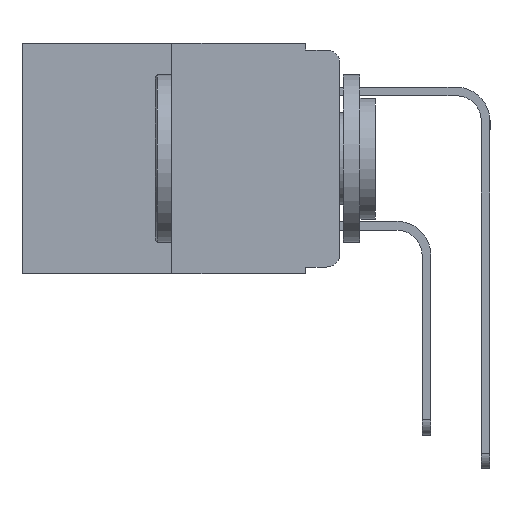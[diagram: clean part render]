
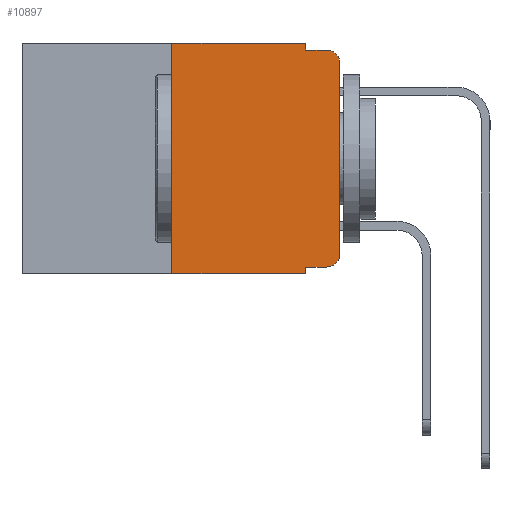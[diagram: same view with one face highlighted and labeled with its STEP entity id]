
A CAD part, left-side view. The second image highlights one B-rep face of the part: STEP entity #10897.
In plain terms, the highlighted planar face has unit normal (-1, 0, 0).
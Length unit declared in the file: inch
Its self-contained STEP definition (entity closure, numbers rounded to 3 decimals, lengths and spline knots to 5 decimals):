
#28 = CARTESIAN_POINT ( 'NONE',  ( 0., 0.051, -0.333 ) ) ;
#94 = VECTOR ( 'NONE', #4774, 39.37008 ) ;
#188 = ORIENTED_EDGE ( 'NONE', *, *, #4034, .T. ) ;
#328 = CARTESIAN_POINT ( 'NONE',  ( 0., 0.473, -0.343 ) ) ;
#418 = CARTESIAN_POINT ( 'NONE',  ( 0., 0.051, -0.01 ) ) ;
#587 = LINE ( 'NONE', #3067, #14895 ) ;
#592 = EDGE_CURVE ( 'NONE', #7211, #11810, #5499, .T. ) ;
#705 = VECTOR ( 'NONE', #10177, 39.37008 ) ;
#743 = CIRCLE ( 'NONE', #8941, 0.02 ) ;
#1153 = AXIS2_PLACEMENT_3D ( 'NONE', #11541, #11527, #11488 ) ;
#1352 = CARTESIAN_POINT ( 'NONE',  ( 0., 0.25, -0.343 ) ) ;
#1393 = VERTEX_POINT ( 'NONE', #7525 ) ;
#1556 = ORIENTED_EDGE ( 'NONE', *, *, #6384, .T. ) ;
#1784 = CARTESIAN_POINT ( 'NONE',  ( 0., 0.051, 0. ) ) ;
#1830 = EDGE_CURVE ( 'NONE', #2861, #8960, #7987, .T. ) ;
#1974 = CARTESIAN_POINT ( 'NONE',  ( 0., 0.25, 0. ) ) ;
#2127 = PLANE ( 'NONE',  #15003 ) ;
#2221 = VECTOR ( 'NONE', #8028, 39.37008 ) ;
#2235 = CARTESIAN_POINT ( 'NONE',  ( 0., 0.051, -0.01 ) ) ;
#2366 = VECTOR ( 'NONE', #13748, 39.37008 ) ;
#2625 = LINE ( 'NONE', #1784, #8626 ) ;
#2861 = VERTEX_POINT ( 'NONE', #1352 ) ;
#2912 = EDGE_CURVE ( 'NONE', #6869, #1393, #8516, .T. ) ;
#2996 = DIRECTION ( 'NONE',  ( 0., 0., -1. ) ) ;
#3067 = CARTESIAN_POINT ( 'NONE',  ( 0., 0.051, 0. ) ) ;
#3073 = ORIENTED_EDGE ( 'NONE', *, *, #1830, .T. ) ;
#3407 = CIRCLE ( 'NONE', #1153, 0.02 ) ;
#3743 = LINE ( 'NONE', #5531, #94 ) ;
#3782 = DIRECTION ( 'NONE',  ( 0., -1., 0. ) ) ;
#3861 = CARTESIAN_POINT ( 'NONE',  ( 0., 0., -0.313 ) ) ;
#4034 = EDGE_CURVE ( 'NONE', #9971, #14086, #6158, .T. ) ;
#4293 = DIRECTION ( 'NONE',  ( 0., 0., -1. ) ) ;
#4603 = DIRECTION ( 'NONE',  ( 0., 0., -1. ) ) ;
#4774 = DIRECTION ( 'NONE',  ( 0., 0., 1. ) ) ;
#5125 = CARTESIAN_POINT ( 'NONE',  ( 0., 0.02, -0.333 ) ) ;
#5277 = CARTESIAN_POINT ( 'NONE',  ( 0., 0.051, 0. ) ) ;
#5281 = CARTESIAN_POINT ( 'NONE',  ( 0., 0.473, 0. ) ) ;
#5420 = EDGE_CURVE ( 'NONE', #6711, #1393, #743, .T. ) ;
#5499 = LINE ( 'NONE', #5281, #2221 ) ;
#5531 = CARTESIAN_POINT ( 'NONE',  ( 0., 0., 0. ) ) ;
#5728 = EDGE_CURVE ( 'NONE', #14086, #8886, #3407, .T. ) ;
#5753 = CARTESIAN_POINT ( 'NONE',  ( 0., 0., -0.03 ) ) ;
#5990 = ORIENTED_EDGE ( 'NONE', *, *, #592, .F. ) ;
#6158 = LINE ( 'NONE', #8670, #14716 ) ;
#6384 = EDGE_CURVE ( 'NONE', #8886, #6711, #3743, .T. ) ;
#6438 = DIRECTION ( 'NONE',  ( 0., 0., -1. ) ) ;
#6455 = DIRECTION ( 'NONE',  ( -1., 0., 0. ) ) ;
#6694 = ORIENTED_EDGE ( 'NONE', *, *, #5728, .T. ) ;
#6711 = VERTEX_POINT ( 'NONE', #5753 ) ;
#6869 = VERTEX_POINT ( 'NONE', #2235 ) ;
#7211 = VERTEX_POINT ( 'NONE', #11182 ) ;
#7319 = CARTESIAN_POINT ( 'NONE',  ( 0., 0.02, -0.03 ) ) ;
#7525 = CARTESIAN_POINT ( 'NONE',  ( 0., 0.02, -0.01 ) ) ;
#7987 = LINE ( 'NONE', #328, #2366 ) ;
#8028 = DIRECTION ( 'NONE',  ( 0., -1., 0. ) ) ;
#8516 = LINE ( 'NONE', #418, #9205 ) ;
#8626 = VECTOR ( 'NONE', #2996, 39.37008 ) ;
#8670 = CARTESIAN_POINT ( 'NONE',  ( 0., 0.051, -0.333 ) ) ;
#8886 = VERTEX_POINT ( 'NONE', #3861 ) ;
#8941 = AXIS2_PLACEMENT_3D ( 'NONE', #7319, #6455, #6438 ) ;
#8960 = VERTEX_POINT ( 'NONE', #10956 ) ;
#9075 = EDGE_CURVE ( 'NONE', #11810, #6869, #587, .T. ) ;
#9205 = VECTOR ( 'NONE', #14351, 39.37008 ) ;
#9379 = ORIENTED_EDGE ( 'NONE', *, *, #14249, .F. ) ;
#9971 = VERTEX_POINT ( 'NONE', #28 ) ;
#10166 = LINE ( 'NONE', #1974, #705 ) ;
#10177 = DIRECTION ( 'NONE',  ( 0., 0., 1. ) ) ;
#10356 = CARTESIAN_POINT ( 'NONE',  ( 0., 0.473, 0. ) ) ;
#10897 = ADVANCED_FACE ( 'NONE', ( #11381 ), #2127, .F. ) ;
#10956 = CARTESIAN_POINT ( 'NONE',  ( 0., 0.051, -0.343 ) ) ;
#11175 = EDGE_LOOP ( 'NONE', ( #1556, #13842, #11231, #14524, #5990, #14884, #3073, #9379, #188, #6694 ) ) ;
#11182 = CARTESIAN_POINT ( 'NONE',  ( 0., 0.25, 0. ) ) ;
#11231 = ORIENTED_EDGE ( 'NONE', *, *, #2912, .F. ) ;
#11381 = FACE_OUTER_BOUND ( 'NONE', #11175, .T. ) ;
#11435 = DIRECTION ( 'NONE',  ( 1., 0., 0. ) ) ;
#11488 = DIRECTION ( 'NONE',  ( 0., 0., -1. ) ) ;
#11527 = DIRECTION ( 'NONE',  ( -1., 0., 0. ) ) ;
#11541 = CARTESIAN_POINT ( 'NONE',  ( 0., 0.02, -0.313 ) ) ;
#11810 = VERTEX_POINT ( 'NONE', #5277 ) ;
#11990 = EDGE_CURVE ( 'NONE', #2861, #7211, #10166, .T. ) ;
#13748 = DIRECTION ( 'NONE',  ( 0., -1., 0. ) ) ;
#13842 = ORIENTED_EDGE ( 'NONE', *, *, #5420, .T. ) ;
#14086 = VERTEX_POINT ( 'NONE', #5125 ) ;
#14249 = EDGE_CURVE ( 'NONE', #9971, #8960, #2625, .T. ) ;
#14351 = DIRECTION ( 'NONE',  ( 0., -1., 0. ) ) ;
#14524 = ORIENTED_EDGE ( 'NONE', *, *, #9075, .F. ) ;
#14716 = VECTOR ( 'NONE', #3782, 39.37008 ) ;
#14884 = ORIENTED_EDGE ( 'NONE', *, *, #11990, .F. ) ;
#14895 = VECTOR ( 'NONE', #4293, 39.37008 ) ;
#15003 = AXIS2_PLACEMENT_3D ( 'NONE', #10356, #11435, #4603 ) ;
